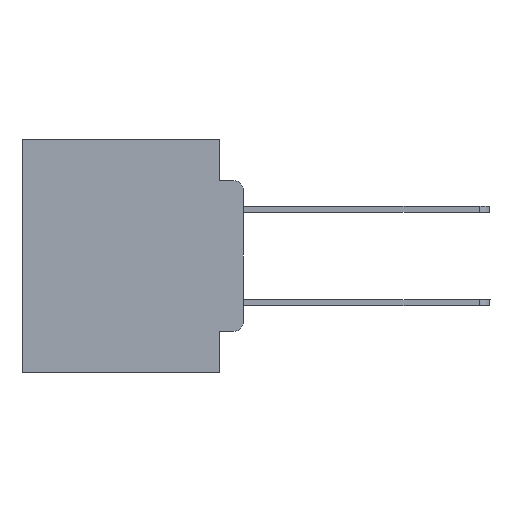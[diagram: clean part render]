
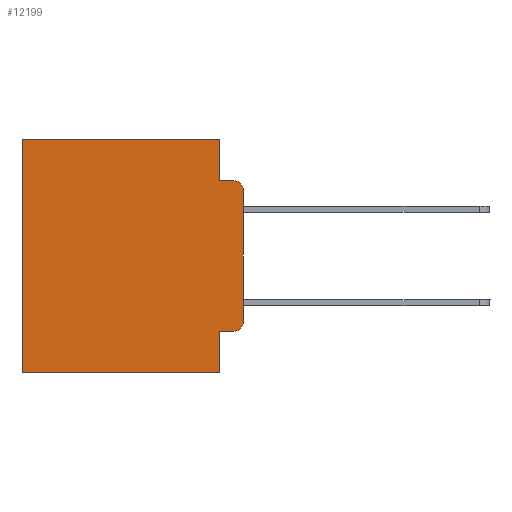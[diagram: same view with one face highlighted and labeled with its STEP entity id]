
A CAD part, left-side view. The second image highlights one B-rep face of the part: STEP entity #12199.
In plain terms, the highlighted planar face has unit normal (-1, 0, 0).
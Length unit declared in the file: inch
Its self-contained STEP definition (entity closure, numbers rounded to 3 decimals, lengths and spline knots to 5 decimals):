
#149 = DIRECTION ( 'NONE',  ( -1., 0., 0. ) ) ;
#733 = VECTOR ( 'NONE', #15359, 39.37008 ) ;
#1562 = LINE ( 'NONE', #19163, #7526 ) ;
#1799 = DIRECTION ( 'NONE',  ( 0., -1., 0. ) ) ;
#1999 = LINE ( 'NONE', #28363, #27914 ) ;
#2308 = AXIS2_PLACEMENT_3D ( 'NONE', #18648, #9852, #22883 ) ;
#3097 = CIRCLE ( 'NONE', #12999, 0.02 ) ;
#3251 = CARTESIAN_POINT ( 'NONE',  ( 0.298, 0.02, -0.4115 ) ) ;
#4015 = CIRCLE ( 'NONE', #20020, 0.02 ) ;
#4375 = EDGE_CURVE ( 'NONE', #25789, #7597, #9119, .T. ) ;
#4822 = CARTESIAN_POINT ( 'NONE',  ( 0.298, 0.051, -0.4115 ) ) ;
#5008 = LINE ( 'NONE', #27416, #28476 ) ;
#5235 = VERTEX_POINT ( 'NONE', #26722 ) ;
#5307 = ORIENTED_EDGE ( 'NONE', *, *, #5737, .T. ) ;
#5480 = LINE ( 'NONE', #6019, #9672 ) ;
#5592 = ORIENTED_EDGE ( 'NONE', *, *, #28545, .F. ) ;
#5716 = ORIENTED_EDGE ( 'NONE', *, *, #18883, .F. ) ;
#5737 = EDGE_CURVE ( 'NONE', #21206, #7142, #3097, .T. ) ;
#5907 = DIRECTION ( 'NONE',  ( 0., -1., 0. ) ) ;
#5963 = CARTESIAN_POINT ( 'NONE',  ( 0.298, 0.051, -0.0885 ) ) ;
#6019 = CARTESIAN_POINT ( 'NONE',  ( 0.298, 0.051, -0.0885 ) ) ;
#6553 = LINE ( 'NONE', #14316, #11725 ) ;
#7020 = VECTOR ( 'NONE', #23615, 39.37008 ) ;
#7142 = VERTEX_POINT ( 'NONE', #12410 ) ;
#7423 = EDGE_CURVE ( 'NONE', #23871, #5235, #16006, .T. ) ;
#7526 = VECTOR ( 'NONE', #27753, 39.37008 ) ;
#7597 = VERTEX_POINT ( 'NONE', #25130 ) ;
#7918 = LINE ( 'NONE', #18889, #13778 ) ;
#8253 = ORIENTED_EDGE ( 'NONE', *, *, #9034, .T. ) ;
#8278 = CARTESIAN_POINT ( 'NONE',  ( 0.298, 0.473, 0. ) ) ;
#8906 = VERTEX_POINT ( 'NONE', #9340 ) ;
#9034 = EDGE_CURVE ( 'NONE', #23871, #21206, #7918, .T. ) ;
#9119 = LINE ( 'NONE', #8278, #7020 ) ;
#9340 = CARTESIAN_POINT ( 'NONE',  ( 0.298, 0., -0.1085 ) ) ;
#9672 = VECTOR ( 'NONE', #1799, 39.37008 ) ;
#9698 = EDGE_CURVE ( 'NONE', #8906, #19689, #4015, .T. ) ;
#9852 = DIRECTION ( 'NONE',  ( 1., 0., 0. ) ) ;
#11089 = EDGE_CURVE ( 'NONE', #21472, #25789, #5008, .T. ) ;
#11725 = VECTOR ( 'NONE', #22851, 39.37008 ) ;
#12199 = ADVANCED_FACE ( 'NONE', ( #27751 ), #13604, .F. ) ;
#12410 = CARTESIAN_POINT ( 'NONE',  ( 0.298, 0., -0.3915 ) ) ;
#12607 = DIRECTION ( 'NONE',  ( 0., 0., -1. ) ) ;
#12999 = AXIS2_PLACEMENT_3D ( 'NONE', #26010, #26118, #28339 ) ;
#13604 = PLANE ( 'NONE',  #2308 ) ;
#13612 = CARTESIAN_POINT ( 'NONE',  ( 0.298, 0.02, -0.0885 ) ) ;
#13778 = VECTOR ( 'NONE', #5907, 39.37008 ) ;
#14225 = DIRECTION ( 'NONE',  ( 0., 1., 0. ) ) ;
#14316 = CARTESIAN_POINT ( 'NONE',  ( 0.298, 0.051, 0. ) ) ;
#14738 = ORIENTED_EDGE ( 'NONE', *, *, #11089, .T. ) ;
#15359 = DIRECTION ( 'NONE',  ( 0., 0., -1. ) ) ;
#15785 = VERTEX_POINT ( 'NONE', #5963 ) ;
#16006 = LINE ( 'NONE', #22070, #733 ) ;
#17974 = CARTESIAN_POINT ( 'NONE',  ( 0.298, 0.051, 0. ) ) ;
#18220 = DIRECTION ( 'NONE',  ( 0., 0., -1. ) ) ;
#18647 = EDGE_LOOP ( 'NONE', ( #5716, #24830, #19418, #5592, #14738, #20064, #21900, #26414, #8253, #5307 ) ) ;
#18648 = CARTESIAN_POINT ( 'NONE',  ( 0.298, 0., 0. ) ) ;
#18744 = CARTESIAN_POINT ( 'NONE',  ( 0.298, 0.473, 0. ) ) ;
#18803 = EDGE_CURVE ( 'NONE', #15785, #19689, #5480, .T. ) ;
#18883 = EDGE_CURVE ( 'NONE', #8906, #7142, #1999, .T. ) ;
#18889 = CARTESIAN_POINT ( 'NONE',  ( 0.298, 0.051, -0.4115 ) ) ;
#19163 = CARTESIAN_POINT ( 'NONE',  ( 0.298, 0., -0.5 ) ) ;
#19418 = ORIENTED_EDGE ( 'NONE', *, *, #18803, .F. ) ;
#19689 = VERTEX_POINT ( 'NONE', #13612 ) ;
#20020 = AXIS2_PLACEMENT_3D ( 'NONE', #24458, #149, #18220 ) ;
#20064 = ORIENTED_EDGE ( 'NONE', *, *, #4375, .T. ) ;
#21206 = VERTEX_POINT ( 'NONE', #3251 ) ;
#21472 = VERTEX_POINT ( 'NONE', #17974 ) ;
#21900 = ORIENTED_EDGE ( 'NONE', *, *, #22388, .F. ) ;
#22070 = CARTESIAN_POINT ( 'NONE',  ( 0.298, 0.051, 0. ) ) ;
#22388 = EDGE_CURVE ( 'NONE', #5235, #7597, #1562, .T. ) ;
#22851 = DIRECTION ( 'NONE',  ( 0., 0., -1. ) ) ;
#22883 = DIRECTION ( 'NONE',  ( 0., 0., -1. ) ) ;
#23615 = DIRECTION ( 'NONE',  ( 0., 0., -1. ) ) ;
#23871 = VERTEX_POINT ( 'NONE', #4822 ) ;
#24458 = CARTESIAN_POINT ( 'NONE',  ( 0.298, 0.02, -0.1085 ) ) ;
#24830 = ORIENTED_EDGE ( 'NONE', *, *, #9698, .T. ) ;
#25130 = CARTESIAN_POINT ( 'NONE',  ( 0.298, 0.473, -0.5 ) ) ;
#25789 = VERTEX_POINT ( 'NONE', #18744 ) ;
#26010 = CARTESIAN_POINT ( 'NONE',  ( 0.298, 0.02, -0.3915 ) ) ;
#26118 = DIRECTION ( 'NONE',  ( -1., 0., 0. ) ) ;
#26414 = ORIENTED_EDGE ( 'NONE', *, *, #7423, .F. ) ;
#26722 = CARTESIAN_POINT ( 'NONE',  ( 0.298, 0.051, -0.5 ) ) ;
#27416 = CARTESIAN_POINT ( 'NONE',  ( 0.298, 0., 0. ) ) ;
#27751 = FACE_OUTER_BOUND ( 'NONE', #18647, .T. ) ;
#27753 = DIRECTION ( 'NONE',  ( 0., 1., 0. ) ) ;
#27914 = VECTOR ( 'NONE', #12607, 39.37008 ) ;
#28339 = DIRECTION ( 'NONE',  ( 0., 0., -1. ) ) ;
#28363 = CARTESIAN_POINT ( 'NONE',  ( 0.298, 0., 0. ) ) ;
#28476 = VECTOR ( 'NONE', #14225, 39.37008 ) ;
#28545 = EDGE_CURVE ( 'NONE', #21472, #15785, #6553, .T. ) ;
